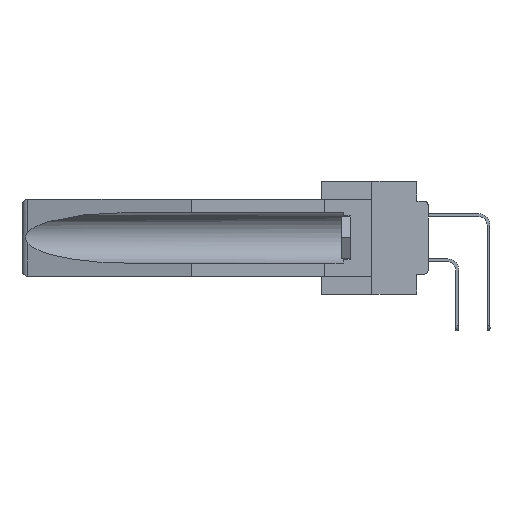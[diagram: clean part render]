
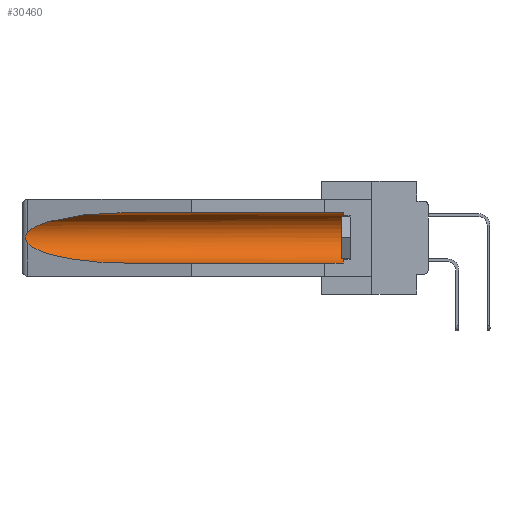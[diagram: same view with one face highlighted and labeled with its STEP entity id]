
A CAD part, left-side view. The second image highlights one B-rep face of the part: STEP entity #30460.
In plain terms, the highlighted cylindrical face has radius 2.857 mm (diameter 5.715 mm), a partial arc.
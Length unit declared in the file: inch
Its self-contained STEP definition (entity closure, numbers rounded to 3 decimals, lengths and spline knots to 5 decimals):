
#337 = AXIS2_PLACEMENT_3D ( 'NONE', #16623, #6341, #31613 ) ;
#338 = DIRECTION ( 'NONE',  ( 0., 1., 0. ) ) ;
#352 = ORIENTED_EDGE ( 'NONE', *, *, #28825, .T. ) ;
#622 = CARTESIAN_POINT ( 'NONE',  ( 0.21114, 1.30732, -0.059 ) ) ;
#973 = VECTOR ( 'NONE', #27267, 39.37008 ) ;
#1393 = LINE ( 'NONE', #1722, #20139 ) ;
#1722 = CARTESIAN_POINT ( 'NONE',  ( 0.155, -0.30754, -0.059 ) ) ;
#2129 = CARTESIAN_POINT ( 'NONE',  ( 0.26537, 1.52718, -0.19328 ) ) ;
#2221 = CARTESIAN_POINT ( 'NONE',  ( 0.2673, 1.53269, -0.17917 ) ) ;
#2597 = VERTEX_POINT ( 'NONE', #32216 ) ;
#2967 = ORIENTED_EDGE ( 'NONE', *, *, #10011, .F. ) ;
#3800 = ORIENTED_EDGE ( 'NONE', *, *, #12341, .T. ) ;
#4381 = DIRECTION ( 'NONE',  ( 0., 1., 0. ) ) ;
#4557 = CARTESIAN_POINT ( 'NONE',  ( 0.2675, 1.53308, -0.17534 ) ) ;
#5964 = VERTEX_POINT ( 'NONE', #24353 ) ;
#6341 = DIRECTION ( 'NONE',  ( 0., -1., 0. ) ) ;
#6948 = ORIENTED_EDGE ( 'NONE', *, *, #19280, .T. ) ;
#7001 = CARTESIAN_POINT ( 'NONE',  ( 0.155, -0.30754, -0.284 ) ) ;
#8671 = CARTESIAN_POINT ( 'NONE',  ( 0.155, 1.07973, -0.284 ) ) ;
#10011 = EDGE_CURVE ( 'NONE', #18716, #20259, #24606, .T. ) ;
#10273 = ORIENTED_EDGE ( 'NONE', *, *, #17137, .T. ) ;
#10584 = CARTESIAN_POINT ( 'NONE',  ( 0.25451, 1.48313, -0.09465 ) ) ;
#11151 = CARTESIAN_POINT ( 'NONE',  ( 0.21114, 1.30732, -0.284 ) ) ;
#11187 = EDGE_CURVE ( 'NONE', #5964, #24985, #1393, .T. ) ;
#12341 = EDGE_CURVE ( 'NONE', #18716, #5964, #28998, .T. ) ;
#13439 = FACE_OUTER_BOUND ( 'NONE', #22015, .T. ) ;
#15001 = CARTESIAN_POINT ( 'NONE',  ( 0.26597, 1.52961, -0.15275 ) ) ;
#16623 = CARTESIAN_POINT ( 'NONE',  ( 0.155, 0.126, -0.1715 ) ) ;
#16924 =( BOUNDED_CURVE ( )  B_SPLINE_CURVE ( 3, ( #31049, #622, #10584, #18733 ),
 .UNSPECIFIED., .F., .F. ) 
 B_SPLINE_CURVE_WITH_KNOTS ( ( 4, 4 ),
 ( 4.71239, 6.08839 ),
 .UNSPECIFIED. ) 
 CURVE ( )  GEOMETRIC_REPRESENTATION_ITEM ( )  RATIONAL_B_SPLINE_CURVE ( ( 1., 0.848, 0.848, 1. ) ) 
 REPRESENTATION_ITEM ( '' )  );
#17137 = EDGE_CURVE ( 'NONE', #2597, #19555, #29712, .T. ) ;
#18236 = CARTESIAN_POINT ( 'NONE',  ( 0.155, 1.07973, -0.059 ) ) ;
#18395 =( BOUNDED_CURVE ( )  B_SPLINE_CURVE ( 3, ( #2129, #24888, #11151, #8671 ),
 .UNSPECIFIED., .F., .F. ) 
 B_SPLINE_CURVE_WITH_KNOTS ( ( 4, 4 ),
 ( 0.1948, 1.5708 ),
 .UNSPECIFIED. ) 
 CURVE ( )  GEOMETRIC_REPRESENTATION_ITEM ( )  RATIONAL_B_SPLINE_CURVE ( ( 1., 0.848, 0.848, 1. ) ) 
 REPRESENTATION_ITEM ( '' )  );
#18716 = VERTEX_POINT ( 'NONE', #31796 ) ;
#18733 = CARTESIAN_POINT ( 'NONE',  ( 0.26537, 1.52718, -0.14972 ) ) ;
#19280 = EDGE_CURVE ( 'NONE', #24985, #2597, #16924, .T. ) ;
#19555 = VERTEX_POINT ( 'NONE', #25537 ) ;
#19675 = CARTESIAN_POINT ( 'NONE',  ( 0.26655, 1.53094, -0.18657 ) ) ;
#19833 = CARTESIAN_POINT ( 'NONE',  ( 0.26537, 1.52718, -0.19328 ) ) ;
#20139 = VECTOR ( 'NONE', #4381, 39.37008 ) ;
#20259 = VERTEX_POINT ( 'NONE', #21931 ) ;
#20444 = CARTESIAN_POINT ( 'NONE',  ( 0.155, -0.30754, -0.1715 ) ) ;
#20928 = DIRECTION ( 'NONE',  ( 0., 0., 1. ) ) ;
#21931 = CARTESIAN_POINT ( 'NONE',  ( 0.155, 1.07973, -0.284 ) ) ;
#22015 = EDGE_LOOP ( 'NONE', ( #6948, #10273, #352, #2967, #3800, #22138 ) ) ;
#22138 = ORIENTED_EDGE ( 'NONE', *, *, #11187, .T. ) ;
#22163 = CARTESIAN_POINT ( 'NONE',  ( 0.26654, 1.53092, -0.15636 ) ) ;
#22489 = CARTESIAN_POINT ( 'NONE',  ( 0.26537, 1.52718, -0.14972 ) ) ;
#22936 = CYLINDRICAL_SURFACE ( 'NONE', #27788, 0.1125 ) ;
#24353 = CARTESIAN_POINT ( 'NONE',  ( 0.155, 0.126, -0.059 ) ) ;
#24606 = LINE ( 'NONE', #7001, #973 ) ;
#24888 = CARTESIAN_POINT ( 'NONE',  ( 0.25451, 1.48313, -0.24835 ) ) ;
#24985 = VERTEX_POINT ( 'NONE', #18236 ) ;
#25537 = CARTESIAN_POINT ( 'NONE',  ( 0.26537, 1.52718, -0.19328 ) ) ;
#27267 = DIRECTION ( 'NONE',  ( 0., 1., 0. ) ) ;
#27652 = CARTESIAN_POINT ( 'NONE',  ( 0.26597, 1.5296, -0.19026 ) ) ;
#27788 = AXIS2_PLACEMENT_3D ( 'NONE', #20444, #338, #20928 ) ;
#28825 = EDGE_CURVE ( 'NONE', #19555, #20259, #18395, .T. ) ;
#28998 = CIRCLE ( 'NONE', #337, 0.1125 ) ;
#29712 = B_SPLINE_CURVE_WITH_KNOTS ( 'NONE', 3,
 ( #22489, #15001, #22163, #30319, #30150, #4557, #2221, #19675, #27652, #19833 ),
 .UNSPECIFIED., .F., .F.,
 ( 4, 2, 2, 2, 4 ),
 ( 0., 0.00029, 0.00058, 0.00087, 0.00117 ),
 .UNSPECIFIED. ) ;
#30150 = CARTESIAN_POINT ( 'NONE',  ( 0.2675, 1.53308, -0.16763 ) ) ;
#30319 = CARTESIAN_POINT ( 'NONE',  ( 0.2673, 1.5327, -0.16383 ) ) ;
#30460 = ADVANCED_FACE ( 'NONE', ( #13439 ), #22936, .F. ) ;
#31049 = CARTESIAN_POINT ( 'NONE',  ( 0.155, 1.07973, -0.059 ) ) ;
#31613 = DIRECTION ( 'NONE',  ( 0., 0., 1. ) ) ;
#31796 = CARTESIAN_POINT ( 'NONE',  ( 0.155, 0.126, -0.284 ) ) ;
#32216 = CARTESIAN_POINT ( 'NONE',  ( 0.26537, 1.52718, -0.14972 ) ) ;
